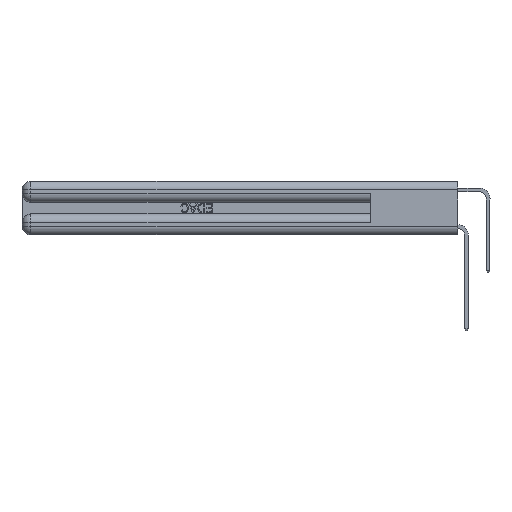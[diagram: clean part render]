
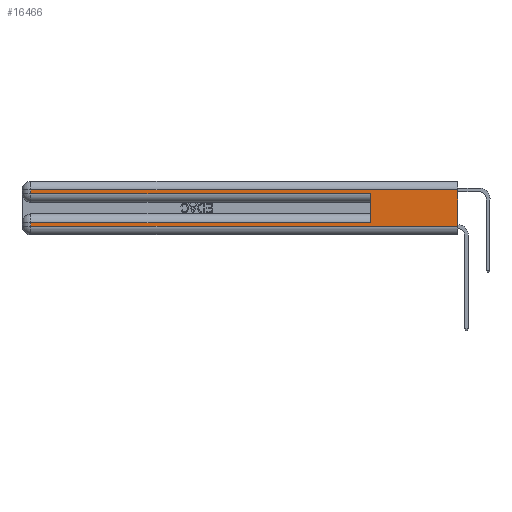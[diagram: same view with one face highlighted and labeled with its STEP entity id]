
A CAD part, left-side view. The second image highlights one B-rep face of the part: STEP entity #16466.
In plain terms, the highlighted planar face has unit normal (-1, 0, 0).
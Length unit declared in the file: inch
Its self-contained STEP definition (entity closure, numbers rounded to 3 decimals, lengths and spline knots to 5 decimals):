
#47 = LINE ( 'NONE', #23684, #3524 ) ;
#50 = DIRECTION ( 'NONE',  ( 0., 0., -1. ) ) ;
#82 = EDGE_CURVE ( 'NONE', #31361, #27182, #185, .T. ) ;
#185 = LINE ( 'NONE', #6395, #26356 ) ;
#2234 = VECTOR ( 'NONE', #19938, 39.37008 ) ;
#3421 = ORIENTED_EDGE ( 'NONE', *, *, #14161, .T. ) ;
#3524 = VECTOR ( 'NONE', #11423, 39.37008 ) ;
#4821 = PLANE ( 'NONE',  #27234 ) ;
#5531 = CARTESIAN_POINT ( 'NONE',  ( 0., 2.94, 0.085 ) ) ;
#5805 = EDGE_CURVE ( 'NONE', #13084, #20977, #30263, .T. ) ;
#6395 = CARTESIAN_POINT ( 'NONE',  ( 0., 0., 0.06 ) ) ;
#6622 = CARTESIAN_POINT ( 'NONE',  ( 0., 2.94, 0.06 ) ) ;
#6927 = VECTOR ( 'NONE', #29806, 39.37008 ) ;
#9025 = DIRECTION ( 'NONE',  ( 0., 1., 0. ) ) ;
#9575 = VERTEX_POINT ( 'NONE', #26487 ) ;
#9795 = ORIENTED_EDGE ( 'NONE', *, *, #30274, .T. ) ;
#10063 = DIRECTION ( 'NONE',  ( 0., -1., 0. ) ) ;
#10387 = VECTOR ( 'NONE', #50, 39.37008 ) ;
#10795 = EDGE_CURVE ( 'NONE', #23688, #28015, #23844, .T. ) ;
#10944 = ORIENTED_EDGE ( 'NONE', *, *, #13397, .F. ) ;
#11257 = CARTESIAN_POINT ( 'NONE',  ( 0., 2.94, 0.31 ) ) ;
#11423 = DIRECTION ( 'NONE',  ( 0., 1., 0. ) ) ;
#11679 = LINE ( 'NONE', #14643, #31304 ) ;
#12013 = LINE ( 'NONE', #31051, #15070 ) ;
#12698 = CARTESIAN_POINT ( 'NONE',  ( 0., 0.6, 0.145 ) ) ;
#13084 = VERTEX_POINT ( 'NONE', #27044 ) ;
#13397 = EDGE_CURVE ( 'NONE', #9575, #27182, #27404, .T. ) ;
#14161 = EDGE_CURVE ( 'NONE', #9575, #23688, #47, .T. ) ;
#14643 = CARTESIAN_POINT ( 'NONE',  ( 0., 0., 0.285 ) ) ;
#15070 = VECTOR ( 'NONE', #9025, 39.37008 ) ;
#16466 = ADVANCED_FACE ( 'NONE', ( #22972 ), #4821, .F. ) ;
#17867 = ORIENTED_EDGE ( 'NONE', *, *, #82, .T. ) ;
#18036 = EDGE_CURVE ( 'NONE', #28015, #20977, #11679, .T. ) ;
#18336 = CARTESIAN_POINT ( 'NONE',  ( 0., 2.94, 0.285 ) ) ;
#18432 = ORIENTED_EDGE ( 'NONE', *, *, #18036, .T. ) ;
#18600 = EDGE_CURVE ( 'NONE', #13084, #28524, #12013, .T. ) ;
#18909 = VECTOR ( 'NONE', #22559, 39.37008 ) ;
#18934 = CARTESIAN_POINT ( 'NONE',  ( 0., 0.6, 0.285 ) ) ;
#19328 = DIRECTION ( 'NONE',  ( 0., 0., -1. ) ) ;
#19938 = DIRECTION ( 'NONE',  ( 0., 0., 1. ) ) ;
#20977 = VERTEX_POINT ( 'NONE', #18934 ) ;
#21125 = DIRECTION ( 'NONE',  ( 0., -1., 0. ) ) ;
#22017 = DIRECTION ( 'NONE',  ( 1., 0., 0. ) ) ;
#22379 = ORIENTED_EDGE ( 'NONE', *, *, #5805, .F. ) ;
#22559 = DIRECTION ( 'NONE',  ( 0., 0., -1. ) ) ;
#22972 = FACE_OUTER_BOUND ( 'NONE', #27449, .T. ) ;
#23684 = CARTESIAN_POINT ( 'NONE',  ( 0., 0., 0.31 ) ) ;
#23688 = VERTEX_POINT ( 'NONE', #11257 ) ;
#23844 = LINE ( 'NONE', #27237, #10387 ) ;
#24769 = CARTESIAN_POINT ( 'NONE',  ( 0., 0., 0.06 ) ) ;
#26356 = VECTOR ( 'NONE', #21125, 39.37008 ) ;
#26487 = CARTESIAN_POINT ( 'NONE',  ( 0., 0., 0.31 ) ) ;
#26572 = LINE ( 'NONE', #29506, #6927 ) ;
#27044 = CARTESIAN_POINT ( 'NONE',  ( 0., 0.6, 0.085 ) ) ;
#27182 = VERTEX_POINT ( 'NONE', #24769 ) ;
#27186 = CARTESIAN_POINT ( 'NONE',  ( 0., 0., 0.37 ) ) ;
#27234 = AXIS2_PLACEMENT_3D ( 'NONE', #29103, #22017, #19328 ) ;
#27237 = CARTESIAN_POINT ( 'NONE',  ( 0., 2.94, 0.37 ) ) ;
#27404 = LINE ( 'NONE', #27186, #18909 ) ;
#27449 = EDGE_LOOP ( 'NONE', ( #10944, #3421, #31374, #18432, #22379, #31235, #9795, #17867 ) ) ;
#28015 = VERTEX_POINT ( 'NONE', #18336 ) ;
#28524 = VERTEX_POINT ( 'NONE', #5531 ) ;
#29103 = CARTESIAN_POINT ( 'NONE',  ( 0., 0., 0.37 ) ) ;
#29506 = CARTESIAN_POINT ( 'NONE',  ( 0., 2.94, 0.37 ) ) ;
#29806 = DIRECTION ( 'NONE',  ( 0., 0., -1. ) ) ;
#30263 = LINE ( 'NONE', #12698, #2234 ) ;
#30274 = EDGE_CURVE ( 'NONE', #28524, #31361, #26572, .T. ) ;
#31051 = CARTESIAN_POINT ( 'NONE',  ( 0., 0., 0.085 ) ) ;
#31235 = ORIENTED_EDGE ( 'NONE', *, *, #18600, .T. ) ;
#31304 = VECTOR ( 'NONE', #10063, 39.37008 ) ;
#31361 = VERTEX_POINT ( 'NONE', #6622 ) ;
#31374 = ORIENTED_EDGE ( 'NONE', *, *, #10795, .T. ) ;
